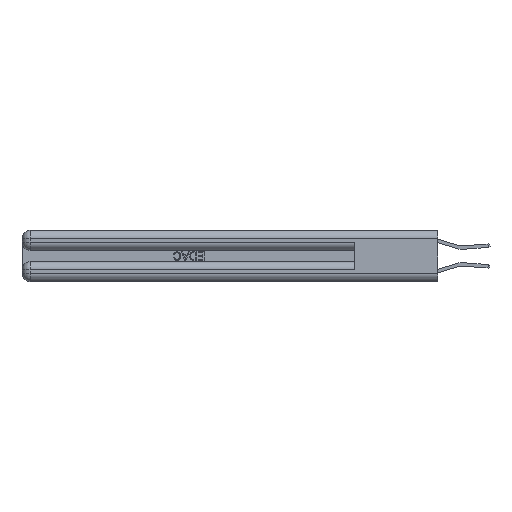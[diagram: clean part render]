
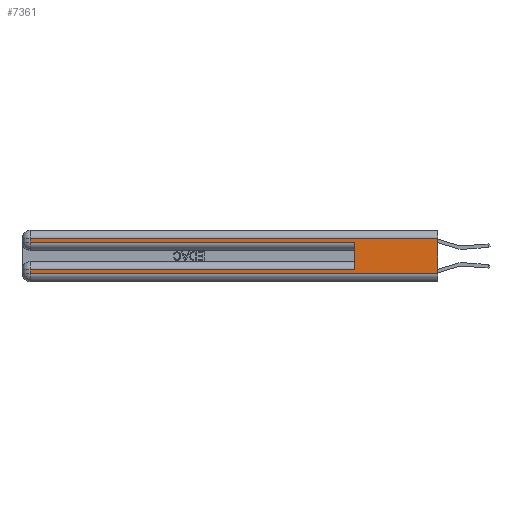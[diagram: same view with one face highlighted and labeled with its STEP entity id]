
A CAD part, left-side view. The second image highlights one B-rep face of the part: STEP entity #7361.
In plain terms, the highlighted planar face has unit normal (-1, 0, 0).
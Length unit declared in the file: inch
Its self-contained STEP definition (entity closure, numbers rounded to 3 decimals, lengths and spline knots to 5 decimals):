
#565 = LINE ( 'NONE', #4373, #2242 ) ;
#651 = DIRECTION ( 'NONE',  ( 1., 0., 0. ) ) ;
#1825 = CARTESIAN_POINT ( 'NONE',  ( 0., 2.94, 0.085 ) ) ;
#2111 = DIRECTION ( 'NONE',  ( 0., 0., -1. ) ) ;
#2242 = VECTOR ( 'NONE', #14855, 39.37008 ) ;
#3195 = CARTESIAN_POINT ( 'NONE',  ( 0., 0.6, 0.285 ) ) ;
#3745 = EDGE_CURVE ( 'NONE', #9490, #29219, #20797, .T. ) ;
#3889 = ORIENTED_EDGE ( 'NONE', *, *, #17540, .T. ) ;
#3896 = DIRECTION ( 'NONE',  ( 0., -1., 0. ) ) ;
#4034 = CARTESIAN_POINT ( 'NONE',  ( 0., 0., 0.37 ) ) ;
#4295 = LINE ( 'NONE', #23205, #5130 ) ;
#4373 = CARTESIAN_POINT ( 'NONE',  ( 0., 0., 0.06 ) ) ;
#4567 = DIRECTION ( 'NONE',  ( 0., 0., -1. ) ) ;
#4855 = ORIENTED_EDGE ( 'NONE', *, *, #12583, .T. ) ;
#5111 = VECTOR ( 'NONE', #6579, 39.37008 ) ;
#5130 = VECTOR ( 'NONE', #2111, 39.37008 ) ;
#6579 = DIRECTION ( 'NONE',  ( 0., 0., -1. ) ) ;
#6791 = EDGE_CURVE ( 'NONE', #9490, #29392, #28887, .T. ) ;
#7361 = ADVANCED_FACE ( 'NONE', ( #25077 ), #16462, .F. ) ;
#8545 = CARTESIAN_POINT ( 'NONE',  ( 0., 0., 0.37 ) ) ;
#9245 = VERTEX_POINT ( 'NONE', #3195 ) ;
#9490 = VERTEX_POINT ( 'NONE', #15889 ) ;
#10191 = CARTESIAN_POINT ( 'NONE',  ( 0., 2.94, 0.31 ) ) ;
#10293 = VECTOR ( 'NONE', #32616, 39.37008 ) ;
#11263 = CARTESIAN_POINT ( 'NONE',  ( 0., 0., 0.085 ) ) ;
#11996 = CARTESIAN_POINT ( 'NONE',  ( 0., 0., 0.285 ) ) ;
#12218 = EDGE_CURVE ( 'NONE', #31529, #9245, #21262, .T. ) ;
#12583 = EDGE_CURVE ( 'NONE', #28528, #29219, #565, .T. ) ;
#13446 = CARTESIAN_POINT ( 'NONE',  ( 0., 0., 0.31 ) ) ;
#14368 = DIRECTION ( 'NONE',  ( 0., 0., 1. ) ) ;
#14494 = ORIENTED_EDGE ( 'NONE', *, *, #27691, .T. ) ;
#14855 = DIRECTION ( 'NONE',  ( 0., -1., 0. ) ) ;
#15589 = ORIENTED_EDGE ( 'NONE', *, *, #3745, .F. ) ;
#15889 = CARTESIAN_POINT ( 'NONE',  ( 0., 0., 0.31 ) ) ;
#15914 = CARTESIAN_POINT ( 'NONE',  ( 0., 0.6, 0.085 ) ) ;
#16462 = PLANE ( 'NONE',  #25889 ) ;
#17540 = EDGE_CURVE ( 'NONE', #24009, #9245, #26808, .T. ) ;
#18045 = EDGE_CURVE ( 'NONE', #31529, #25462, #23867, .T. ) ;
#18991 = DIRECTION ( 'NONE',  ( 0., 0., -1. ) ) ;
#20668 = CARTESIAN_POINT ( 'NONE',  ( 0., 2.94, 0.06 ) ) ;
#20797 = LINE ( 'NONE', #4034, #5111 ) ;
#21262 = LINE ( 'NONE', #24875, #31671 ) ;
#21300 = ORIENTED_EDGE ( 'NONE', *, *, #18045, .T. ) ;
#21540 = VECTOR ( 'NONE', #4567, 39.37008 ) ;
#21620 = ORIENTED_EDGE ( 'NONE', *, *, #31943, .T. ) ;
#21859 = CARTESIAN_POINT ( 'NONE',  ( 0., 2.94, 0.285 ) ) ;
#22155 = CARTESIAN_POINT ( 'NONE',  ( 0., 0., 0.06 ) ) ;
#22630 = VECTOR ( 'NONE', #26592, 39.37008 ) ;
#22650 = CARTESIAN_POINT ( 'NONE',  ( 0., 2.94, 0.37 ) ) ;
#23205 = CARTESIAN_POINT ( 'NONE',  ( 0., 2.94, 0.37 ) ) ;
#23867 = LINE ( 'NONE', #11263, #10293 ) ;
#24009 = VERTEX_POINT ( 'NONE', #21859 ) ;
#24739 = VECTOR ( 'NONE', #3896, 39.37008 ) ;
#24875 = CARTESIAN_POINT ( 'NONE',  ( 0., 0.6, 0.145 ) ) ;
#25077 = FACE_OUTER_BOUND ( 'NONE', #30001, .T. ) ;
#25462 = VERTEX_POINT ( 'NONE', #1825 ) ;
#25889 = AXIS2_PLACEMENT_3D ( 'NONE', #8545, #651, #18991 ) ;
#26592 = DIRECTION ( 'NONE',  ( 0., 1., 0. ) ) ;
#26808 = LINE ( 'NONE', #11996, #24739 ) ;
#26945 = LINE ( 'NONE', #22650, #21540 ) ;
#27691 = EDGE_CURVE ( 'NONE', #29392, #24009, #26945, .T. ) ;
#28528 = VERTEX_POINT ( 'NONE', #20668 ) ;
#28887 = LINE ( 'NONE', #13446, #22630 ) ;
#28981 = ORIENTED_EDGE ( 'NONE', *, *, #6791, .T. ) ;
#29219 = VERTEX_POINT ( 'NONE', #22155 ) ;
#29392 = VERTEX_POINT ( 'NONE', #10191 ) ;
#30001 = EDGE_LOOP ( 'NONE', ( #15589, #28981, #14494, #3889, #33468, #21300, #21620, #4855 ) ) ;
#31529 = VERTEX_POINT ( 'NONE', #15914 ) ;
#31671 = VECTOR ( 'NONE', #14368, 39.37008 ) ;
#31943 = EDGE_CURVE ( 'NONE', #25462, #28528, #4295, .T. ) ;
#32616 = DIRECTION ( 'NONE',  ( 0., 1., 0. ) ) ;
#33468 = ORIENTED_EDGE ( 'NONE', *, *, #12218, .F. ) ;
